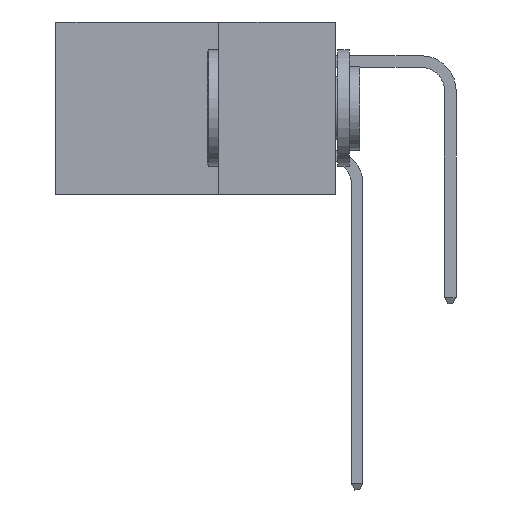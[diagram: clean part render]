
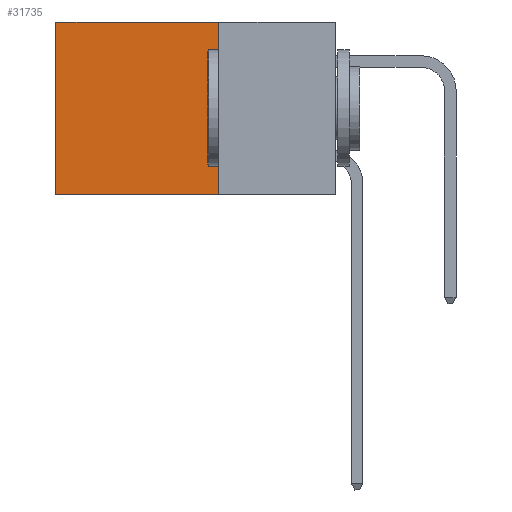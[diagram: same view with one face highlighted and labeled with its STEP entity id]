
A CAD part, left-side view. The second image highlights one B-rep face of the part: STEP entity #31735.
In plain terms, the highlighted planar face has unit normal (-1, 0, 0).
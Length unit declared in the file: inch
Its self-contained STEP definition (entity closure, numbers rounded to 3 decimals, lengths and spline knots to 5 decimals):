
#73 = DIRECTION ( 'NONE',  ( 0., 1., 0. ) ) ;
#2980 = EDGE_LOOP ( 'NONE', ( #24308, #19865, #11942, #20059 ) ) ;
#4051 = VERTEX_POINT ( 'NONE', #33169 ) ;
#4207 = EDGE_CURVE ( 'NONE', #8490, #12124, #9665, .T. ) ;
#5556 = DIRECTION ( 'NONE',  ( 0., 0., -1. ) ) ;
#7371 = CARTESIAN_POINT ( 'NONE',  ( 0.2875, 0.25, -0.37 ) ) ;
#8490 = VERTEX_POINT ( 'NONE', #12371 ) ;
#8781 = VECTOR ( 'NONE', #73, 39.37008 ) ;
#9633 = CARTESIAN_POINT ( 'NONE',  ( 0.2875, 0.6, 0. ) ) ;
#9665 = LINE ( 'NONE', #11295, #16130 ) ;
#10197 = AXIS2_PLACEMENT_3D ( 'NONE', #21593, #40396, #5556 ) ;
#10819 = LINE ( 'NONE', #28270, #37093 ) ;
#11295 = CARTESIAN_POINT ( 'NONE',  ( 0.2875, 0.25, 0. ) ) ;
#11942 = ORIENTED_EDGE ( 'NONE', *, *, #31151, .F. ) ;
#12124 = VERTEX_POINT ( 'NONE', #9633 ) ;
#12310 = DIRECTION ( 'NONE',  ( 0., 0., -1. ) ) ;
#12371 = CARTESIAN_POINT ( 'NONE',  ( 0.2875, 0.25, 0. ) ) ;
#13385 = DIRECTION ( 'NONE',  ( 0., 1., 0. ) ) ;
#16130 = VECTOR ( 'NONE', #13385, 39.37008 ) ;
#16251 = EDGE_CURVE ( 'NONE', #26920, #4051, #29667, .T. ) ;
#16536 = FACE_OUTER_BOUND ( 'NONE', #2980, .T. ) ;
#18568 = LINE ( 'NONE', #31179, #30462 ) ;
#19865 = ORIENTED_EDGE ( 'NONE', *, *, #16251, .F. ) ;
#20059 = ORIENTED_EDGE ( 'NONE', *, *, #4207, .T. ) ;
#21593 = CARTESIAN_POINT ( 'NONE',  ( 0.2875, 0.25, 0. ) ) ;
#24308 = ORIENTED_EDGE ( 'NONE', *, *, #37982, .T. ) ;
#24992 = DIRECTION ( 'NONE',  ( 0., 0., -1. ) ) ;
#26920 = VERTEX_POINT ( 'NONE', #7371 ) ;
#27973 = PLANE ( 'NONE',  #10197 ) ;
#28270 = CARTESIAN_POINT ( 'NONE',  ( 0.2875, 0.6, 0. ) ) ;
#29667 = LINE ( 'NONE', #38122, #8781 ) ;
#30462 = VECTOR ( 'NONE', #24992, 39.37008 ) ;
#31151 = EDGE_CURVE ( 'NONE', #8490, #26920, #18568, .T. ) ;
#31179 = CARTESIAN_POINT ( 'NONE',  ( 0.2875, 0.25, 0. ) ) ;
#31735 = ADVANCED_FACE ( 'NONE', ( #16536 ), #27973, .F. ) ;
#33169 = CARTESIAN_POINT ( 'NONE',  ( 0.2875, 0.6, -0.37 ) ) ;
#37093 = VECTOR ( 'NONE', #12310, 39.37008 ) ;
#37982 = EDGE_CURVE ( 'NONE', #12124, #4051, #10819, .T. ) ;
#38122 = CARTESIAN_POINT ( 'NONE',  ( 0.2875, 0.25, -0.37 ) ) ;
#40396 = DIRECTION ( 'NONE',  ( 1., 0., 0. ) ) ;
